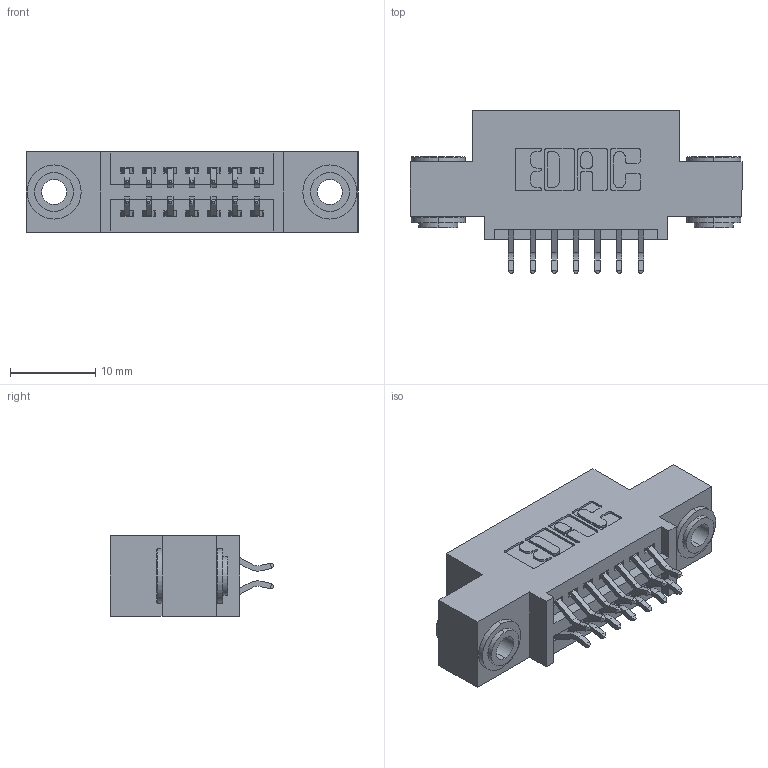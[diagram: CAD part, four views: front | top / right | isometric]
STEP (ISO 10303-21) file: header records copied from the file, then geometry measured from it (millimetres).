
FILE_DESCRIPTION (( 'STEP AP203' ), '1' );
FILE_NAME ('395-014-556-503.STEP', '2018-11-06T01:28:25', ( '' ), ( '' ), 'SwSTEP 2.0', 'SolidWorks 2016', '' );
FILE_SCHEMA (( 'CONFIG_CONTROL_DESIGN' ));
Length unit declared in the file: inch
Products named in the file (4): 395-014-556-503; 345-292-001_556 Tail; 345 Part_0.110 Offset - 0.156 Dia-TH; 345-250-002_345-250-002-102
Assembly tree (17 placements, depth 2):
  395-014-556-503
    345 Part_0.110 Offset - 0.156 Dia-TH
    345-292-001_556 Tail  x14
    345-250-002_345-250-002-102  x2
Bounding box: 38.99 x 19.24 x 9.4 mm (x, y, z)
Volume: 3408 mm3; surface area: 4645.2 mm2
Topology: 17 solids, 17 shells, 952 faces, 2767 edges, 1822 vertices
Faces by surface type: plane 612, cylinder 332, cone 8
Entity records: 11206 total; most frequent: CARTESIAN_POINT 1903, ORIENTED_EDGE 1818, DIRECTION 1739, EDGE_CURVE 909, LINE 717, VECTOR 717, VERTEX_POINT 602, AXIS2_PLACEMENT_3D 511
